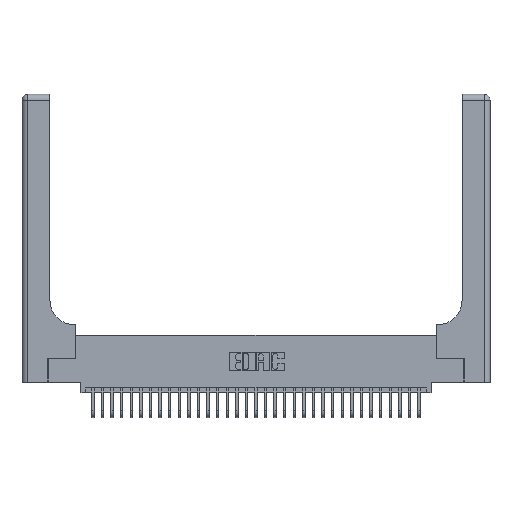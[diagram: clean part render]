
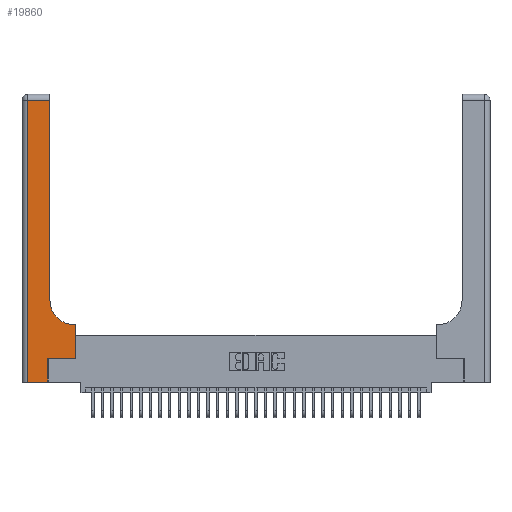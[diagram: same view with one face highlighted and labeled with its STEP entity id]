
A CAD part, top view. The second image highlights one B-rep face of the part: STEP entity #19860.
In plain terms, the highlighted planar face has unit normal (0, 0, 1).
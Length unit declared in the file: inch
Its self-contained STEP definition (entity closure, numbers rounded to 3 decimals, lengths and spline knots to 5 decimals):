
#597 = VERTEX_POINT ( 'NONE', #21961 ) ;
#917 = ORIENTED_EDGE ( 'NONE', *, *, #28564, .T. ) ;
#1564 = VERTEX_POINT ( 'NONE', #17566 ) ;
#1740 = VERTEX_POINT ( 'NONE', #15510 ) ;
#1827 = EDGE_CURVE ( 'NONE', #20131, #28372, #33617, .T. ) ;
#2366 = LINE ( 'NONE', #7676, #30593 ) ;
#2569 = DIRECTION ( 'NONE',  ( -1., 0., 0. ) ) ;
#2675 = CARTESIAN_POINT ( 'NONE',  ( 0., 2.94, 0.37 ) ) ;
#4984 = DIRECTION ( 'NONE',  ( 0., 0., -1. ) ) ;
#5099 = DIRECTION ( 'NONE',  ( 1., 0., 0. ) ) ;
#5128 = CARTESIAN_POINT ( 'NONE',  ( 0.269, 0., 0.37 ) ) ;
#5244 = EDGE_LOOP ( 'NONE', ( #23747, #16244, #26952, #917, #13769, #9907, #12647, #6714, #12514 ) ) ;
#5426 = VECTOR ( 'NONE', #10657, 39.37008 ) ;
#6497 = CARTESIAN_POINT ( 'NONE',  ( 0.2915, 0.85, 0.37 ) ) ;
#6714 = ORIENTED_EDGE ( 'NONE', *, *, #25892, .T. ) ;
#7676 = CARTESIAN_POINT ( 'NONE',  ( 0.269, 0.25, 0.37 ) ) ;
#7784 = EDGE_CURVE ( 'NONE', #597, #27416, #33793, .T. ) ;
#8011 = CARTESIAN_POINT ( 'NONE',  ( 0.2915, 3., 0.37 ) ) ;
#8532 = FACE_OUTER_BOUND ( 'NONE', #5244, .T. ) ;
#8835 = CARTESIAN_POINT ( 'NONE',  ( 0.269, 0., 0.37 ) ) ;
#9736 = EDGE_CURVE ( 'NONE', #28372, #1740, #31102, .T. ) ;
#9907 = ORIENTED_EDGE ( 'NONE', *, *, #10737, .T. ) ;
#10254 = VECTOR ( 'NONE', #5099, 39.37008 ) ;
#10452 = DIRECTION ( 'NONE',  ( 1., 0., 0. ) ) ;
#10657 = DIRECTION ( 'NONE',  ( 0., 1., 0. ) ) ;
#10737 = EDGE_CURVE ( 'NONE', #12505, #597, #2366, .T. ) ;
#11109 = LINE ( 'NONE', #18686, #10254 ) ;
#11212 = LINE ( 'NONE', #32330, #33002 ) ;
#11314 = LINE ( 'NONE', #30914, #32238 ) ;
#11916 = DIRECTION ( 'NONE',  ( -1., 0., 0. ) ) ;
#11994 = VECTOR ( 'NONE', #15416, 39.37008 ) ;
#12505 = VERTEX_POINT ( 'NONE', #31706 ) ;
#12514 = ORIENTED_EDGE ( 'NONE', *, *, #33845, .T. ) ;
#12647 = ORIENTED_EDGE ( 'NONE', *, *, #7784, .T. ) ;
#13769 = ORIENTED_EDGE ( 'NONE', *, *, #23994, .T. ) ;
#14241 = LINE ( 'NONE', #8835, #27931 ) ;
#15130 = AXIS2_PLACEMENT_3D ( 'NONE', #21342, #4984, #24090 ) ;
#15416 = DIRECTION ( 'NONE',  ( 0., 1., 0. ) ) ;
#15510 = CARTESIAN_POINT ( 'NONE',  ( 0.06, 2.94, 0.37 ) ) ;
#15953 = DIRECTION ( 'NONE',  ( 0., -1., 0. ) ) ;
#16164 = CARTESIAN_POINT ( 'NONE',  ( 0., 3., 0.37 ) ) ;
#16244 = ORIENTED_EDGE ( 'NONE', *, *, #9736, .T. ) ;
#16322 = VERTEX_POINT ( 'NONE', #25180 ) ;
#17566 = CARTESIAN_POINT ( 'NONE',  ( 0.06, 0., 0.37 ) ) ;
#18686 = CARTESIAN_POINT ( 'NONE',  ( 0., 0., 0.37 ) ) ;
#18912 = DIRECTION ( 'NONE',  ( 0., 0., -1. ) ) ;
#19860 = ADVANCED_FACE ( 'NONE', ( #8532 ), #32543, .F. ) ;
#20131 = VERTEX_POINT ( 'NONE', #6497 ) ;
#20592 = AXIS2_PLACEMENT_3D ( 'NONE', #16164, #18912, #2569 ) ;
#21059 = VERTEX_POINT ( 'NONE', #5128 ) ;
#21342 = CARTESIAN_POINT ( 'NONE',  ( 0.5415, 0.85, 0.37 ) ) ;
#21961 = CARTESIAN_POINT ( 'NONE',  ( 0.5585, 0.25, 0.37 ) ) ;
#23683 = CIRCLE ( 'NONE', #15130, 0.25 ) ;
#23747 = ORIENTED_EDGE ( 'NONE', *, *, #1827, .T. ) ;
#23816 = VECTOR ( 'NONE', #30029, 39.37008 ) ;
#23994 = EDGE_CURVE ( 'NONE', #21059, #12505, #14241, .T. ) ;
#24090 = DIRECTION ( 'NONE',  ( 1., 0., 0. ) ) ;
#25180 = CARTESIAN_POINT ( 'NONE',  ( 0.5415, 0.6, 0.37 ) ) ;
#25193 = DIRECTION ( 'NONE',  ( 0., 1., 0. ) ) ;
#25892 = EDGE_CURVE ( 'NONE', #27416, #16322, #11314, .T. ) ;
#26615 = CARTESIAN_POINT ( 'NONE',  ( 0.5585, 0.6, 0.37 ) ) ;
#26952 = ORIENTED_EDGE ( 'NONE', *, *, #34959, .T. ) ;
#27416 = VERTEX_POINT ( 'NONE', #26615 ) ;
#27931 = VECTOR ( 'NONE', #25193, 39.37008 ) ;
#28372 = VERTEX_POINT ( 'NONE', #28996 ) ;
#28564 = EDGE_CURVE ( 'NONE', #1564, #21059, #11109, .T. ) ;
#28996 = CARTESIAN_POINT ( 'NONE',  ( 0.2915, 2.94, 0.37 ) ) ;
#29077 = CARTESIAN_POINT ( 'NONE',  ( 0.5585, 0.25, 0.37 ) ) ;
#30029 = DIRECTION ( 'NONE',  ( -1., 0., 0. ) ) ;
#30593 = VECTOR ( 'NONE', #10452, 39.37008 ) ;
#30914 = CARTESIAN_POINT ( 'NONE',  ( 0.2915, 0.6, 0.37 ) ) ;
#31102 = LINE ( 'NONE', #2675, #23816 ) ;
#31706 = CARTESIAN_POINT ( 'NONE',  ( 0.269, 0.25, 0.37 ) ) ;
#32238 = VECTOR ( 'NONE', #11916, 39.37008 ) ;
#32330 = CARTESIAN_POINT ( 'NONE',  ( 0.06, 3., 0.37 ) ) ;
#32543 = PLANE ( 'NONE',  #20592 ) ;
#33002 = VECTOR ( 'NONE', #15953, 39.37008 ) ;
#33617 = LINE ( 'NONE', #8011, #5426 ) ;
#33793 = LINE ( 'NONE', #29077, #11994 ) ;
#33845 = EDGE_CURVE ( 'NONE', #16322, #20131, #23683, .T. ) ;
#34959 = EDGE_CURVE ( 'NONE', #1740, #1564, #11212, .T. ) ;
